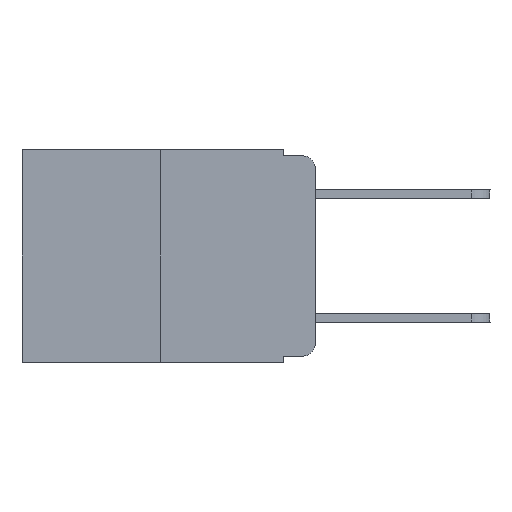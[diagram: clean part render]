
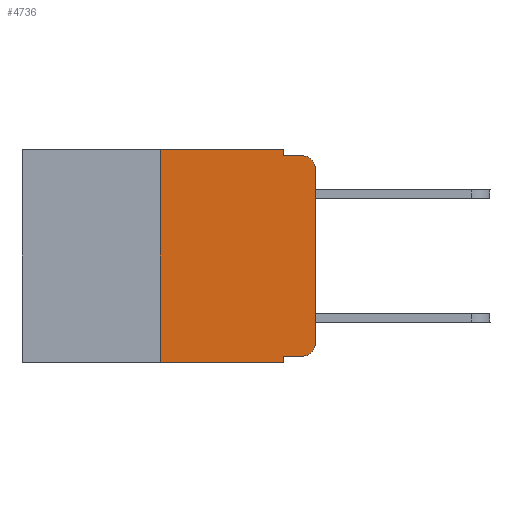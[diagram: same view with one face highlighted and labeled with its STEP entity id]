
A CAD part, left-side view. The second image highlights one B-rep face of the part: STEP entity #4736.
In plain terms, the highlighted planar face has unit normal (-1, 0, 0).
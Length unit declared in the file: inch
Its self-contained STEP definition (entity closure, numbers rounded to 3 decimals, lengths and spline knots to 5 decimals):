
#35 = CARTESIAN_POINT ( 'NONE',  ( 0., 0.25, 0. ) ) ;
#79 = ORIENTED_EDGE ( 'NONE', *, *, #7516, .T. ) ;
#164 = DIRECTION ( 'NONE',  ( 0., -1., 0. ) ) ;
#172 = EDGE_CURVE ( 'NONE', #2650, #1183, #3425, .T. ) ;
#362 = VERTEX_POINT ( 'NONE', #11025 ) ;
#512 = EDGE_LOOP ( 'NONE', ( #7166, #5333, #7317, #8497, #1589, #8965, #2087, #548, #79, #858 ) ) ;
#548 = ORIENTED_EDGE ( 'NONE', *, *, #172, .F. ) ;
#579 = DIRECTION ( 'NONE',  ( 0., 0., -1. ) ) ;
#858 = ORIENTED_EDGE ( 'NONE', *, *, #2793, .T. ) ;
#944 = VERTEX_POINT ( 'NONE', #4051 ) ;
#1074 = CARTESIAN_POINT ( 'NONE',  ( 0., 0.051, -0.343 ) ) ;
#1183 = VERTEX_POINT ( 'NONE', #1074 ) ;
#1263 = VECTOR ( 'NONE', #6301, 39.37008 ) ;
#1357 = CARTESIAN_POINT ( 'NONE',  ( 0., 0.051, -0.01 ) ) ;
#1473 = CIRCLE ( 'NONE', #2923, 0.02 ) ;
#1480 = DIRECTION ( 'NONE',  ( 0., -1., 0. ) ) ;
#1497 = CARTESIAN_POINT ( 'NONE',  ( 0., 0., 0. ) ) ;
#1589 = ORIENTED_EDGE ( 'NONE', *, *, #6739, .F. ) ;
#1597 = EDGE_CURVE ( 'NONE', #944, #10548, #7047, .T. ) ;
#1643 = LINE ( 'NONE', #1700, #8068 ) ;
#1647 = DIRECTION ( 'NONE',  ( 0., 0., -1. ) ) ;
#1700 = CARTESIAN_POINT ( 'NONE',  ( 0., 0.473, -0.343 ) ) ;
#1701 = LINE ( 'NONE', #35, #6569 ) ;
#1702 = FACE_OUTER_BOUND ( 'NONE', #512, .T. ) ;
#2087 = ORIENTED_EDGE ( 'NONE', *, *, #2847, .T. ) ;
#2086 = DIRECTION ( 'NONE',  ( 0., -1., 0. ) ) ;
#2130 = VECTOR ( 'NONE', #2086, 39.37008 ) ;
#2131 = DIRECTION ( 'NONE',  ( -1., 0., 0. ) ) ;
#2190 = LINE ( 'NONE', #1497, #11197 ) ;
#2509 = DIRECTION ( 'NONE',  ( -1., 0., 0. ) ) ;
#2650 = VERTEX_POINT ( 'NONE', #6486 ) ;
#2721 = VERTEX_POINT ( 'NONE', #8407 ) ;
#2793 = EDGE_CURVE ( 'NONE', #2721, #7559, #9715, .T. ) ;
#2847 = EDGE_CURVE ( 'NONE', #8336, #1183, #1643, .T. ) ;
#2923 = AXIS2_PLACEMENT_3D ( 'NONE', #5712, #2131, #579 ) ;
#3071 = CARTESIAN_POINT ( 'NONE',  ( 0., 0.051, -0.333 ) ) ;
#3425 = LINE ( 'NONE', #5136, #5783 ) ;
#3653 = VECTOR ( 'NONE', #9217, 39.37008 ) ;
#4051 = CARTESIAN_POINT ( 'NONE',  ( 0., 0.051, 0. ) ) ;
#4447 = LINE ( 'NONE', #3071, #7292 ) ;
#4662 = CARTESIAN_POINT ( 'NONE',  ( 0., 0.051, -0.01 ) ) ;
#4736 = ADVANCED_FACE ( 'NONE', ( #1702 ), #11289, .F. ) ;
#5136 = CARTESIAN_POINT ( 'NONE',  ( 0., 0.051, 0. ) ) ;
#5333 = ORIENTED_EDGE ( 'NONE', *, *, #7237, .T. ) ;
#5369 = DIRECTION ( 'NONE',  ( 0., 0., -1. ) ) ;
#5452 = CARTESIAN_POINT ( 'NONE',  ( 0., 0.051, 0. ) ) ;
#5712 = CARTESIAN_POINT ( 'NONE',  ( 0., 0.02, -0.03 ) ) ;
#5783 = VECTOR ( 'NONE', #5369, 39.37008 ) ;
#5874 = DIRECTION ( 'NONE',  ( 0., 0., 1. ) ) ;
#5967 = DIRECTION ( 'NONE',  ( 0., 0., 1. ) ) ;
#6301 = DIRECTION ( 'NONE',  ( 0., 0., -1. ) ) ;
#6486 = CARTESIAN_POINT ( 'NONE',  ( 0., 0.051, -0.333 ) ) ;
#6569 = VECTOR ( 'NONE', #5967, 39.37008 ) ;
#6739 = EDGE_CURVE ( 'NONE', #362, #944, #8097, .T. ) ;
#6752 = LINE ( 'NONE', #1357, #3653 ) ;
#6760 = CARTESIAN_POINT ( 'NONE',  ( 0., 0.02, -0.313 ) ) ;
#6849 = AXIS2_PLACEMENT_3D ( 'NONE', #6998, #10391, #1647 ) ;
#6998 = CARTESIAN_POINT ( 'NONE',  ( 0., 0.473, 0. ) ) ;
#7047 = LINE ( 'NONE', #5452, #1263 ) ;
#7166 = ORIENTED_EDGE ( 'NONE', *, *, #8400, .T. ) ;
#7237 = EDGE_CURVE ( 'NONE', #7594, #7978, #1473, .T. ) ;
#7292 = VECTOR ( 'NONE', #164, 39.37008 ) ;
#7317 = ORIENTED_EDGE ( 'NONE', *, *, #7600, .F. ) ;
#7516 = EDGE_CURVE ( 'NONE', #2650, #2721, #4447, .T. ) ;
#7559 = VERTEX_POINT ( 'NONE', #10692 ) ;
#7594 = VERTEX_POINT ( 'NONE', #8826 ) ;
#7600 = EDGE_CURVE ( 'NONE', #10548, #7978, #6752, .T. ) ;
#7957 = CARTESIAN_POINT ( 'NONE',  ( 0., 0.25, -0.343 ) ) ;
#7978 = VERTEX_POINT ( 'NONE', #9811 ) ;
#8068 = VECTOR ( 'NONE', #1480, 39.37008 ) ;
#8097 = LINE ( 'NONE', #9920, #2130 ) ;
#8336 = VERTEX_POINT ( 'NONE', #7957 ) ;
#8400 = EDGE_CURVE ( 'NONE', #7559, #7594, #2190, .T. ) ;
#8407 = CARTESIAN_POINT ( 'NONE',  ( 0., 0.02, -0.333 ) ) ;
#8497 = ORIENTED_EDGE ( 'NONE', *, *, #1597, .F. ) ;
#8826 = CARTESIAN_POINT ( 'NONE',  ( 0., 0., -0.03 ) ) ;
#8965 = ORIENTED_EDGE ( 'NONE', *, *, #10380, .F. ) ;
#9217 = DIRECTION ( 'NONE',  ( 0., -1., 0. ) ) ;
#9715 = CIRCLE ( 'NONE', #11149, 0.02 ) ;
#9811 = CARTESIAN_POINT ( 'NONE',  ( 0., 0.02, -0.01 ) ) ;
#9920 = CARTESIAN_POINT ( 'NONE',  ( 0., 0.473, 0. ) ) ;
#10380 = EDGE_CURVE ( 'NONE', #8336, #362, #1701, .T. ) ;
#10391 = DIRECTION ( 'NONE',  ( 1., 0., 0. ) ) ;
#10548 = VERTEX_POINT ( 'NONE', #4662 ) ;
#10692 = CARTESIAN_POINT ( 'NONE',  ( 0., 0., -0.313 ) ) ;
#11025 = CARTESIAN_POINT ( 'NONE',  ( 0., 0.25, 0. ) ) ;
#11149 = AXIS2_PLACEMENT_3D ( 'NONE', #6760, #2509, #11285 ) ;
#11197 = VECTOR ( 'NONE', #5874, 39.37008 ) ;
#11285 = DIRECTION ( 'NONE',  ( 0., 0., -1. ) ) ;
#11289 = PLANE ( 'NONE',  #6849 ) ;
